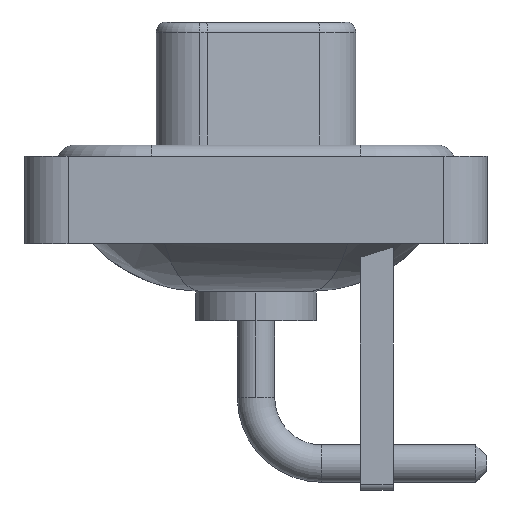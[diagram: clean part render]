
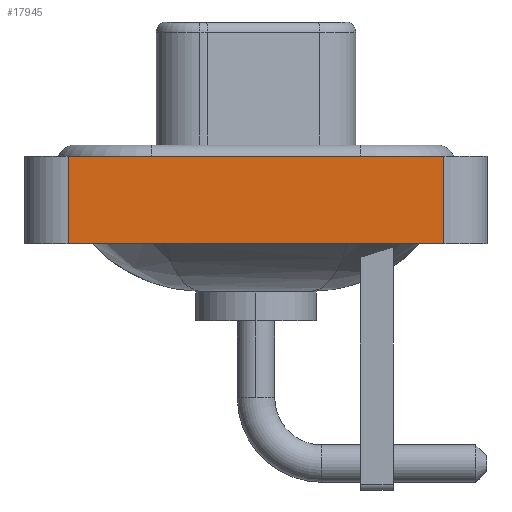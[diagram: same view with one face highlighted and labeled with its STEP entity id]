
A CAD part, left-side view. The second image highlights one B-rep face of the part: STEP entity #17945.
In plain terms, the highlighted planar face has unit normal (-1, 0, 0).
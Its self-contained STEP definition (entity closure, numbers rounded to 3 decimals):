
#112 = VECTOR ( 'NONE', #15804, 1000. ) ;
#433 = ORIENTED_EDGE ( 'NONE', *, *, #2686, .F. ) ;
#599 = EDGE_CURVE ( 'NONE', #4984, #5795, #3941, .T. ) ;
#1641 = CARTESIAN_POINT ( 'NONE',  ( -7.25, -8.55, 0.4 ) ) ;
#1825 = DIRECTION ( 'NONE',  ( -1., 0., 0. ) ) ;
#2621 = CARTESIAN_POINT ( 'NONE',  ( -7.25, -8.55, 0.4 ) ) ;
#2686 = EDGE_CURVE ( 'NONE', #8521, #4984, #18648, .T. ) ;
#3061 = ORIENTED_EDGE ( 'NONE', *, *, #16405, .T. ) ;
#3112 = LINE ( 'NONE', #14576, #3936 ) ;
#3449 = FACE_OUTER_BOUND ( 'NONE', #16132, .T. ) ;
#3936 = VECTOR ( 'NONE', #17526, 1000. ) ;
#3941 = LINE ( 'NONE', #2621, #112 ) ;
#4723 = CARTESIAN_POINT ( 'NONE',  ( -7.25, 8.55, 0.4 ) ) ;
#4984 = VERTEX_POINT ( 'NONE', #4723 ) ;
#5795 = VERTEX_POINT ( 'NONE', #1641 ) ;
#8521 = VERTEX_POINT ( 'NONE', #12071 ) ;
#8630 = CARTESIAN_POINT ( 'NONE',  ( -7.25, -8.55, -3.6 ) ) ;
#9190 = DIRECTION ( 'NONE',  ( 0., 0., 1. ) ) ;
#9376 = PLANE ( 'NONE',  #13331 ) ;
#9725 = VERTEX_POINT ( 'NONE', #15691 ) ;
#9782 = DIRECTION ( 'NONE',  ( 0., 0., 1. ) ) ;
#10311 = DIRECTION ( 'NONE',  ( 0., -1., 0. ) ) ;
#12071 = CARTESIAN_POINT ( 'NONE',  ( -7.25, 8.55, -3.6 ) ) ;
#12696 = CARTESIAN_POINT ( 'NONE',  ( -7.25, 8.55, -3.6 ) ) ;
#13317 = VECTOR ( 'NONE', #10311, 1000. ) ;
#13331 = AXIS2_PLACEMENT_3D ( 'NONE', #14831, #1825, #9190 ) ;
#13869 = ORIENTED_EDGE ( 'NONE', *, *, #599, .F. ) ;
#14462 = EDGE_CURVE ( 'NONE', #9725, #5795, #3112, .T. ) ;
#14576 = CARTESIAN_POINT ( 'NONE',  ( -7.25, -8.55, -3.6 ) ) ;
#14831 = CARTESIAN_POINT ( 'NONE',  ( -7.25, -8.55, -3.6 ) ) ;
#15664 = ORIENTED_EDGE ( 'NONE', *, *, #14462, .T. ) ;
#15691 = CARTESIAN_POINT ( 'NONE',  ( -7.25, -8.55, -3.6 ) ) ;
#15804 = DIRECTION ( 'NONE',  ( 0., -1., 0. ) ) ;
#16074 = LINE ( 'NONE', #8630, #13317 ) ;
#16132 = EDGE_LOOP ( 'NONE', ( #15664, #13869, #433, #3061 ) ) ;
#16405 = EDGE_CURVE ( 'NONE', #8521, #9725, #16074, .T. ) ;
#16946 = VECTOR ( 'NONE', #9782, 1000. ) ;
#17526 = DIRECTION ( 'NONE',  ( 0., 0., 1. ) ) ;
#17945 = ADVANCED_FACE ( 'NONE', ( #3449 ), #9376, .T. ) ;
#18648 = LINE ( 'NONE', #12696, #16946 ) ;
